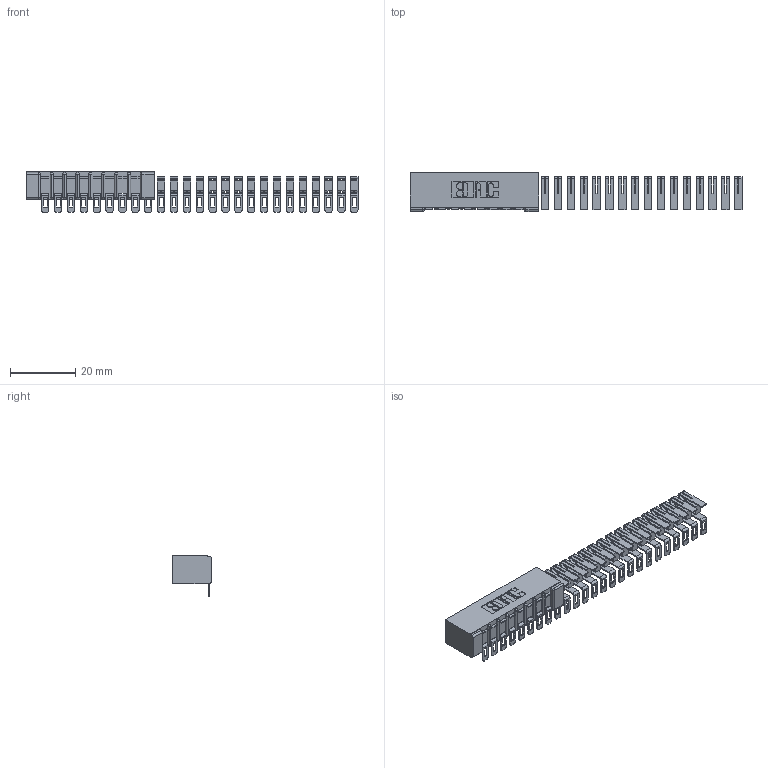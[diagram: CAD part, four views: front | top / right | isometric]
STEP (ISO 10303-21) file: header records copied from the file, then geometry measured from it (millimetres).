
FILE_DESCRIPTION (( 'STEP AP203' ), '1' );
FILE_NAME ('357-025-554-101.STEP', '2018-08-09T02:14:08', ( '' ), ( '' ), 'SwSTEP 2.0', 'SolidWorks 2016', '' );
FILE_SCHEMA (( 'CONFIG_CONTROL_DESIGN' ));
Length unit declared in the file: inch
Products named in the file (3): 307 Part_No Mounting Lugs; 307-290-002_554; 357-025-554-101
Assembly tree (26 placements, depth 2):
  357-025-554-101
    307 Part_No Mounting Lugs
    307-290-002_554  x25
Bounding box: 102.15 x 12.01 x 12.52 mm (x, y, z)
Volume: 3348.5 mm3; surface area: 8788.7 mm2
Topology: 26 solids, 26 shells, 1804 faces, 5536 edges, 3664 vertices
Faces by surface type: plane 1012, cylinder 774, sphere 18
Entity records: 12281 total; most frequent: CARTESIAN_POINT 1991, DIRECTION 1972, ORIENTED_EDGE 1964, EDGE_CURVE 982, LINE 730, VECTOR 730, VERTEX_POINT 640, AXIS2_PLACEMENT_3D 621
